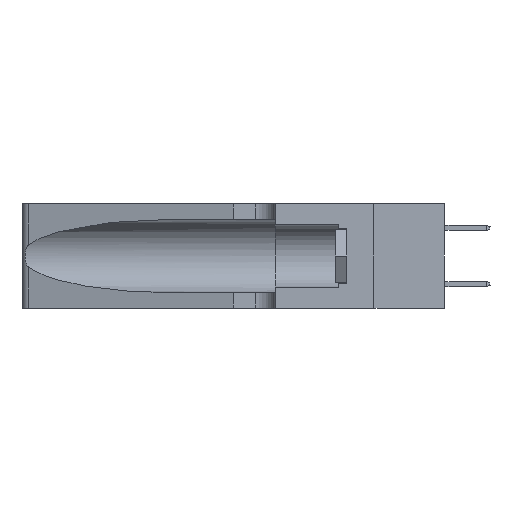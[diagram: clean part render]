
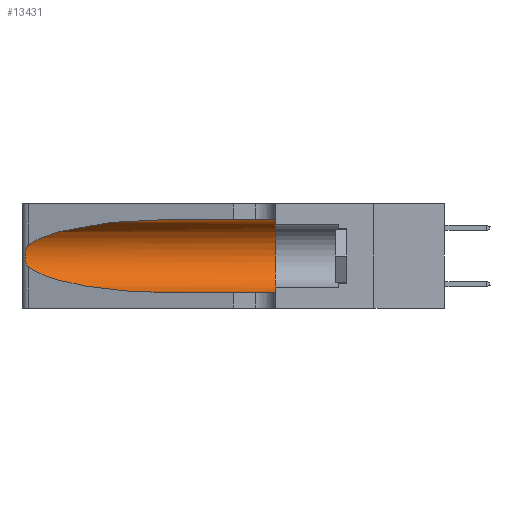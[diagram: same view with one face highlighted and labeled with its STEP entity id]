
A CAD part, left-side view. The second image highlights one B-rep face of the part: STEP entity #13431.
In plain terms, the highlighted cylindrical face has radius 3.308 mm (diameter 6.617 mm), a partial arc.
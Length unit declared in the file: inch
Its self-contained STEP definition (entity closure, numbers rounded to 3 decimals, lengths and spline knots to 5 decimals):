
#111 = EDGE_CURVE ( 'NONE', #14624, #2556, #2939, .T. ) ;
#133 = CARTESIAN_POINT ( 'NONE',  ( 0.26075, 1.23896, 0.19203 ) ) ;
#217 = CARTESIAN_POINT ( 'NONE',  ( 0.26018, 1.23835, 0.19895 ) ) ;
#409 =( BOUNDED_CURVE ( )  B_SPLINE_CURVE ( 3, ( #1796, #3757, #17115, #5702 ),
 .UNSPECIFIED., .F., .F. ) 
 B_SPLINE_CURVE_WITH_KNOTS ( ( 4, 4 ),
 ( 1.5708, 2.84003 ),
 .UNSPECIFIED. ) 
 CURVE ( )  GEOMETRIC_REPRESENTATION_ITEM ( )  RATIONAL_B_SPLINE_CURVE ( ( 1., 0.87, 0.87, 1. ) ) 
 REPRESENTATION_ITEM ( '' )  );
#464 = CARTESIAN_POINT ( 'NONE',  ( 0.25854, 1.2359, 0.20912 ) ) ;
#537 = LINE ( 'NONE', #3650, #14695 ) ;
#672 = CARTESIAN_POINT ( 'NONE',  ( 0.25487, 1.22718, 0.14631 ) ) ;
#881 = CARTESIAN_POINT ( 'NONE',  ( 0.25787, 1.23484, 0.2124 ) ) ;
#902 = EDGE_CURVE ( 'NONE', #2556, #2831, #2754, .T. ) ;
#1308 = DIRECTION ( 'NONE',  ( 0., -1., 0. ) ) ;
#1443 = CARTESIAN_POINT ( 'NONE',  ( 0.1305, 0.72297, 0.05475 ) ) ;
#1608 = CARTESIAN_POINT ( 'NONE',  ( 0.25487, 1.22718, 0.14631 ) ) ;
#1796 = CARTESIAN_POINT ( 'NONE',  ( 0.1305, 0.72297, 0.31525 ) ) ;
#1877 = AXIS2_PLACEMENT_3D ( 'NONE', #3314, #18682, #20581 ) ;
#1996 = ORIENTED_EDGE ( 'NONE', *, *, #8315, .F. ) ;
#2349 = CYLINDRICAL_SURFACE ( 'NONE', #1877, 0.13025 ) ;
#2420 = ORIENTED_EDGE ( 'NONE', *, *, #902, .T. ) ;
#2556 = VERTEX_POINT ( 'NONE', #672 ) ;
#2754 =( BOUNDED_CURVE ( )  B_SPLINE_CURVE ( 3, ( #1608, #13133, #3584, #16925 ),
 .UNSPECIFIED., .F., .F. ) 
 B_SPLINE_CURVE_WITH_KNOTS ( ( 4, 4 ),
 ( 3.44316, 4.71239 ),
 .UNSPECIFIED. ) 
 CURVE ( )  GEOMETRIC_REPRESENTATION_ITEM ( )  RATIONAL_B_SPLINE_CURVE ( ( 1., 0.87, 0.87, 1. ) ) 
 REPRESENTATION_ITEM ( '' )  );
#2808 = CARTESIAN_POINT ( 'NONE',  ( 0.25856, 1.23593, 0.16098 ) ) ;
#2831 = VERTEX_POINT ( 'NONE', #1443 ) ;
#2939 = B_SPLINE_CURVE_WITH_KNOTS ( 'NONE', 3,
 ( #3374, #3467, #3619, #881, #464, #217, #133, #5506, #5315, #2808, #21590, #24711, #11683, #11570 ),
 .UNSPECIFIED., .F., .F.,
 ( 4, 2, 2, 2, 2, 2, 4 ),
 ( 0., 0.00027, 0.00053, 0.00107, 0.0016, 0.00187, 0.00214 ),
 .UNSPECIFIED. ) ;
#3314 = CARTESIAN_POINT ( 'NONE',  ( 0.1305, 1.61858, 0.185 ) ) ;
#3374 = CARTESIAN_POINT ( 'NONE',  ( 0.25487, 1.22718, 0.22369 ) ) ;
#3467 = CARTESIAN_POINT ( 'NONE',  ( 0.25555, 1.22994, 0.2215 ) ) ;
#3584 = CARTESIAN_POINT ( 'NONE',  ( 0.18966, 0.96281, 0.05475 ) ) ;
#3619 = CARTESIAN_POINT ( 'NONE',  ( 0.25639, 1.23184, 0.21858 ) ) ;
#3635 = ORIENTED_EDGE ( 'NONE', *, *, #23877, .T. ) ;
#3650 = CARTESIAN_POINT ( 'NONE',  ( 0.1305, 1.61858, 0.05475 ) ) ;
#3757 = CARTESIAN_POINT ( 'NONE',  ( 0.18966, 0.96281, 0.31525 ) ) ;
#4186 = FACE_OUTER_BOUND ( 'NONE', #18730, .T. ) ;
#5255 = ORIENTED_EDGE ( 'NONE', *, *, #8308, .F. ) ;
#5315 = CARTESIAN_POINT ( 'NONE',  ( 0.26017, 1.23833, 0.17102 ) ) ;
#5506 = CARTESIAN_POINT ( 'NONE',  ( 0.26075, 1.23896, 0.178 ) ) ;
#5702 = CARTESIAN_POINT ( 'NONE',  ( 0.25487, 1.22718, 0.22369 ) ) ;
#6725 = ORIENTED_EDGE ( 'NONE', *, *, #111, .T. ) ;
#7003 = AXIS2_PLACEMENT_3D ( 'NONE', #11030, #24300, #12922 ) ;
#7512 = CARTESIAN_POINT ( 'NONE',  ( 0.1305, 0.35, 0.05475 ) ) ;
#8308 = EDGE_CURVE ( 'NONE', #12994, #9606, #17104, .T. ) ;
#8315 = EDGE_CURVE ( 'NONE', #9606, #15455, #23352, .T. ) ;
#9059 = CARTESIAN_POINT ( 'NONE',  ( 0.1305, 0.35, 0.31525 ) ) ;
#9606 = VERTEX_POINT ( 'NONE', #9059 ) ;
#11030 = CARTESIAN_POINT ( 'NONE',  ( 0.1305, 0.35, 0.185 ) ) ;
#11570 = CARTESIAN_POINT ( 'NONE',  ( 0.25487, 1.22718, 0.14631 ) ) ;
#11683 = CARTESIAN_POINT ( 'NONE',  ( 0.25555, 1.22993, 0.14849 ) ) ;
#12845 = CARTESIAN_POINT ( 'NONE',  ( 0.1305, 1.61858, 0.31525 ) ) ;
#12922 = DIRECTION ( 'NONE',  ( 0., 0., 1. ) ) ;
#12994 = VERTEX_POINT ( 'NONE', #24292 ) ;
#13133 = CARTESIAN_POINT ( 'NONE',  ( 0.2373, 1.15595, 0.08982 ) ) ;
#13263 = VECTOR ( 'NONE', #1308, 39.37008 ) ;
#13431 = ADVANCED_FACE ( 'NONE', ( #4186 ), #2349, .F. ) ;
#14624 = VERTEX_POINT ( 'NONE', #22356 ) ;
#14695 = VECTOR ( 'NONE', #15098, 39.37008 ) ;
#15098 = DIRECTION ( 'NONE',  ( 0., -1., 0. ) ) ;
#15455 = VERTEX_POINT ( 'NONE', #7512 ) ;
#16925 = CARTESIAN_POINT ( 'NONE',  ( 0.1305, 0.72297, 0.05475 ) ) ;
#17104 = LINE ( 'NONE', #12845, #13263 ) ;
#17115 = CARTESIAN_POINT ( 'NONE',  ( 0.2373, 1.15595, 0.28018 ) ) ;
#18682 = DIRECTION ( 'NONE',  ( 0., -1., 0. ) ) ;
#18730 = EDGE_LOOP ( 'NONE', ( #24385, #6725, #2420, #3635, #1996, #5255 ) ) ;
#20581 = DIRECTION ( 'NONE',  ( 0., 0., -1. ) ) ;
#21590 = CARTESIAN_POINT ( 'NONE',  ( 0.25789, 1.23486, 0.15765 ) ) ;
#22356 = CARTESIAN_POINT ( 'NONE',  ( 0.25487, 1.22718, 0.22369 ) ) ;
#23266 = EDGE_CURVE ( 'NONE', #12994, #14624, #409, .T. ) ;
#23352 = CIRCLE ( 'NONE', #7003, 0.13025 ) ;
#23877 = EDGE_CURVE ( 'NONE', #2831, #15455, #537, .T. ) ;
#24292 = CARTESIAN_POINT ( 'NONE',  ( 0.1305, 0.72297, 0.31525 ) ) ;
#24300 = DIRECTION ( 'NONE',  ( 0., 1., 0. ) ) ;
#24385 = ORIENTED_EDGE ( 'NONE', *, *, #23266, .T. ) ;
#24711 = CARTESIAN_POINT ( 'NONE',  ( 0.25639, 1.23186, 0.15144 ) ) ;
